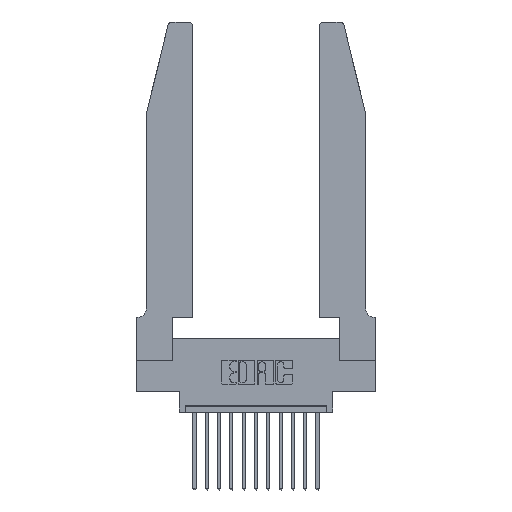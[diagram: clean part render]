
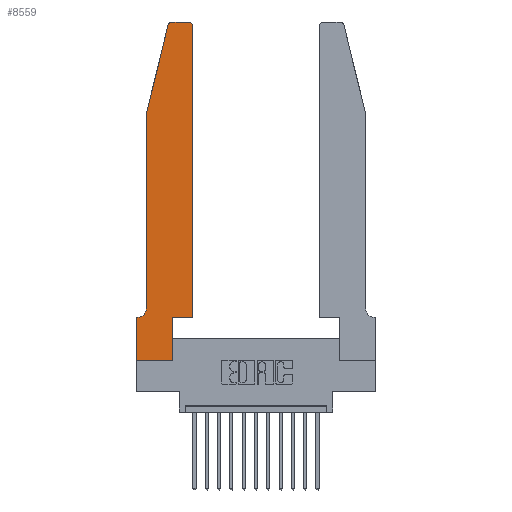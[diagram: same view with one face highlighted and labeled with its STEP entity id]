
A CAD part, top view. The second image highlights one B-rep face of the part: STEP entity #8559.
In plain terms, the highlighted planar face has unit normal (0, 0, 1).
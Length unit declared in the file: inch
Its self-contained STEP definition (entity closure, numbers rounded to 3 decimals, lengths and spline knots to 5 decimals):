
#15 = CARTESIAN_POINT ( 'NONE',  ( 0.284, 2.72, 0.37 ) ) ;
#98 = EDGE_CURVE ( 'NONE', #3640, #5576, #1424, .T. ) ;
#131 = CARTESIAN_POINT ( 'NONE',  ( 0.4205, 2.75, 0.37 ) ) ;
#372 = EDGE_CURVE ( 'NONE', #16188, #11859, #4175, .T. ) ;
#377 = VERTEX_POINT ( 'NONE', #12451 ) ;
#752 = VERTEX_POINT ( 'NONE', #6730 ) ;
#1032 = ORIENTED_EDGE ( 'NONE', *, *, #12836, .T. ) ;
#1050 = VERTEX_POINT ( 'NONE', #131 ) ;
#1280 = LINE ( 'NONE', #6325, #11583 ) ;
#1424 = LINE ( 'NONE', #2904, #10872 ) ;
#1516 = VECTOR ( 'NONE', #6982, 39.37008 ) ;
#1929 = VECTOR ( 'NONE', #7489, 39.37008 ) ;
#2074 = DIRECTION ( 'NONE',  ( -1., 0., 0. ) ) ;
#2272 = VERTEX_POINT ( 'NONE', #11652 ) ;
#2437 = ORIENTED_EDGE ( 'NONE', *, *, #16346, .T. ) ;
#2904 = CARTESIAN_POINT ( 'NONE',  ( 0.2865, 0.35, 0.37 ) ) ;
#2932 = VECTOR ( 'NONE', #8440, 39.37008 ) ;
#2939 = ORIENTED_EDGE ( 'NONE', *, *, #98, .T. ) ;
#3248 = CARTESIAN_POINT ( 'NONE',  ( 0.4205, 2.72, 0.37 ) ) ;
#3429 = CARTESIAN_POINT ( 'NONE',  ( 0.4505, 2.72, 0.37 ) ) ;
#3500 = AXIS2_PLACEMENT_3D ( 'NONE', #5152, #3837, #14472 ) ;
#3562 = CIRCLE ( 'NONE', #6745, 0.03 ) ;
#3640 = VERTEX_POINT ( 'NONE', #10690 ) ;
#3777 = PLANE ( 'NONE',  #3500 ) ;
#3837 = DIRECTION ( 'NONE',  ( 0., 0., 1. ) ) ;
#3936 = CARTESIAN_POINT ( 'NONE',  ( 0.4505, 0.35, 0.37 ) ) ;
#3955 = CARTESIAN_POINT ( 'NONE',  ( 0.0755, 0.35, 0.37 ) ) ;
#4101 = VECTOR ( 'NONE', #16048, 39.37008 ) ;
#4103 = DIRECTION ( 'NONE',  ( 0., 1., 0. ) ) ;
#4175 = LINE ( 'NONE', #10273, #13791 ) ;
#4218 = DIRECTION ( 'NONE',  ( 1., 0., 0. ) ) ;
#4651 = EDGE_CURVE ( 'NONE', #1050, #16870, #1280, .T. ) ;
#4814 = EDGE_CURVE ( 'NONE', #11859, #1050, #11993, .T. ) ;
#4825 = CARTESIAN_POINT ( 'NONE',  ( 0., 0., 0.37 ) ) ;
#5021 = ORIENTED_EDGE ( 'NONE', *, *, #15580, .T. ) ;
#5152 = CARTESIAN_POINT ( 'NONE',  ( 0., 0.35, 0.37 ) ) ;
#5181 = AXIS2_PLACEMENT_3D ( 'NONE', #3248, #11461, #12594 ) ;
#5476 = ORIENTED_EDGE ( 'NONE', *, *, #372, .T. ) ;
#5576 = VERTEX_POINT ( 'NONE', #7071 ) ;
#6325 = CARTESIAN_POINT ( 'NONE',  ( 0.2605, 2.75, 0.37 ) ) ;
#6730 = CARTESIAN_POINT ( 'NONE',  ( 0., 0.35, 0.37 ) ) ;
#6745 = AXIS2_PLACEMENT_3D ( 'NONE', #15, #13317, #4218 ) ;
#6751 = VERTEX_POINT ( 'NONE', #12473 ) ;
#6781 = EDGE_CURVE ( 'NONE', #16870, #9671, #3562, .T. ) ;
#6982 = DIRECTION ( 'NONE',  ( -0.239, -0.971, 0. ) ) ;
#6998 = EDGE_CURVE ( 'NONE', #5576, #16188, #15489, .T. ) ;
#7071 = CARTESIAN_POINT ( 'NONE',  ( 0.2865, 0.35, 0.37 ) ) ;
#7489 = DIRECTION ( 'NONE',  ( 0., -1., 0. ) ) ;
#8029 = ORIENTED_EDGE ( 'NONE', *, *, #4814, .T. ) ;
#8223 = ORIENTED_EDGE ( 'NONE', *, *, #12809, .T. ) ;
#8285 = EDGE_CURVE ( 'NONE', #15474, #377, #13187, .T. ) ;
#8298 = CARTESIAN_POINT ( 'NONE',  ( 0.0755, 2., 0.37 ) ) ;
#8440 = DIRECTION ( 'NONE',  ( 1., 0., 0. ) ) ;
#8476 = EDGE_LOOP ( 'NONE', ( #16193, #10960, #2437, #5021, #10085, #8223, #14405, #1032, #2939, #10064, #5476, #8029 ) ) ;
#8559 = ADVANCED_FACE ( 'NONE', ( #10615 ), #3777, .T. ) ;
#8797 = VECTOR ( 'NONE', #11063, 39.37008 ) ;
#9229 = CARTESIAN_POINT ( 'NONE',  ( 0.25487, 2.72718, 0.37 ) ) ;
#9671 = VERTEX_POINT ( 'NONE', #9229 ) ;
#9783 = CARTESIAN_POINT ( 'NONE',  ( 0.284, 2.75, 0.37 ) ) ;
#9834 = CARTESIAN_POINT ( 'NONE',  ( 0.4505, 0.35, 0.37 ) ) ;
#10059 = LINE ( 'NONE', #3955, #8797 ) ;
#10064 = ORIENTED_EDGE ( 'NONE', *, *, #6998, .T. ) ;
#10085 = ORIENTED_EDGE ( 'NONE', *, *, #8285, .T. ) ;
#10273 = CARTESIAN_POINT ( 'NONE',  ( 0.4505, 0.35, 0.37 ) ) ;
#10369 = CARTESIAN_POINT ( 'NONE',  ( 0.0055, 0.42, 0.37 ) ) ;
#10481 = DIRECTION ( 'NONE',  ( 0., 0., -1. ) ) ;
#10615 = FACE_OUTER_BOUND ( 'NONE', #8476, .T. ) ;
#10690 = CARTESIAN_POINT ( 'NONE',  ( 0.2865, 0., 0.37 ) ) ;
#10872 = VECTOR ( 'NONE', #4103, 39.37008 ) ;
#10960 = ORIENTED_EDGE ( 'NONE', *, *, #6781, .T. ) ;
#11063 = DIRECTION ( 'NONE',  ( -1., 0., 0. ) ) ;
#11122 = CARTESIAN_POINT ( 'NONE',  ( 0., 0., 0.37 ) ) ;
#11184 = LINE ( 'NONE', #8298, #1516 ) ;
#11461 = DIRECTION ( 'NONE',  ( 0., 0., 1. ) ) ;
#11583 = VECTOR ( 'NONE', #2074, 39.37008 ) ;
#11652 = CARTESIAN_POINT ( 'NONE',  ( 0., 0., 0.37 ) ) ;
#11859 = VERTEX_POINT ( 'NONE', #3429 ) ;
#11993 = CIRCLE ( 'NONE', #5181, 0.03 ) ;
#12062 = LINE ( 'NONE', #13227, #4101 ) ;
#12451 = CARTESIAN_POINT ( 'NONE',  ( 0.0055, 0.35, 0.37 ) ) ;
#12473 = CARTESIAN_POINT ( 'NONE',  ( 0.0755, 2., 0.37 ) ) ;
#12574 = DIRECTION ( 'NONE',  ( 1., 0., 0. ) ) ;
#12594 = DIRECTION ( 'NONE',  ( 1., 0., 0. ) ) ;
#12809 = EDGE_CURVE ( 'NONE', #377, #752, #10059, .T. ) ;
#12836 = EDGE_CURVE ( 'NONE', #2272, #3640, #16516, .T. ) ;
#13187 = CIRCLE ( 'NONE', #14909, 0.07 ) ;
#13204 = DIRECTION ( 'NONE',  ( -1., 0., 0. ) ) ;
#13227 = CARTESIAN_POINT ( 'NONE',  ( 0.0755, 2., 0.37 ) ) ;
#13317 = DIRECTION ( 'NONE',  ( 0., 0., 1. ) ) ;
#13505 = LINE ( 'NONE', #4825, #1929 ) ;
#13791 = VECTOR ( 'NONE', #14659, 39.37008 ) ;
#14405 = ORIENTED_EDGE ( 'NONE', *, *, #16570, .T. ) ;
#14472 = DIRECTION ( 'NONE',  ( 1., 0., 0. ) ) ;
#14659 = DIRECTION ( 'NONE',  ( 0., 1., 0. ) ) ;
#14909 = AXIS2_PLACEMENT_3D ( 'NONE', #10369, #10481, #13204 ) ;
#15474 = VERTEX_POINT ( 'NONE', #15779 ) ;
#15489 = LINE ( 'NONE', #9834, #16288 ) ;
#15580 = EDGE_CURVE ( 'NONE', #6751, #15474, #12062, .T. ) ;
#15779 = CARTESIAN_POINT ( 'NONE',  ( 0.0755, 0.42, 0.37 ) ) ;
#16048 = DIRECTION ( 'NONE',  ( 0., -1., 0. ) ) ;
#16188 = VERTEX_POINT ( 'NONE', #3936 ) ;
#16193 = ORIENTED_EDGE ( 'NONE', *, *, #4651, .T. ) ;
#16288 = VECTOR ( 'NONE', #12574, 39.37008 ) ;
#16346 = EDGE_CURVE ( 'NONE', #9671, #6751, #11184, .T. ) ;
#16516 = LINE ( 'NONE', #11122, #2932 ) ;
#16570 = EDGE_CURVE ( 'NONE', #752, #2272, #13505, .T. ) ;
#16870 = VERTEX_POINT ( 'NONE', #9783 ) ;
